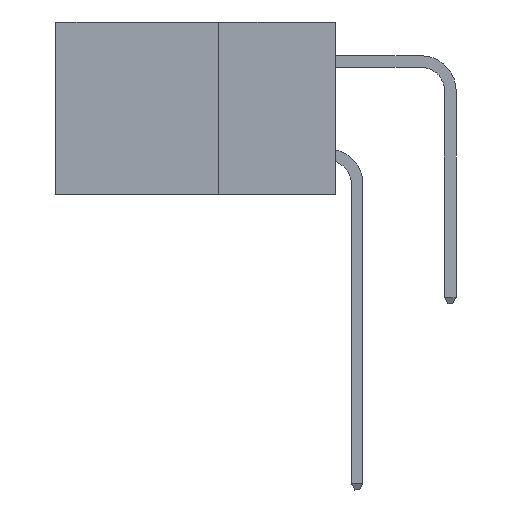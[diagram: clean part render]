
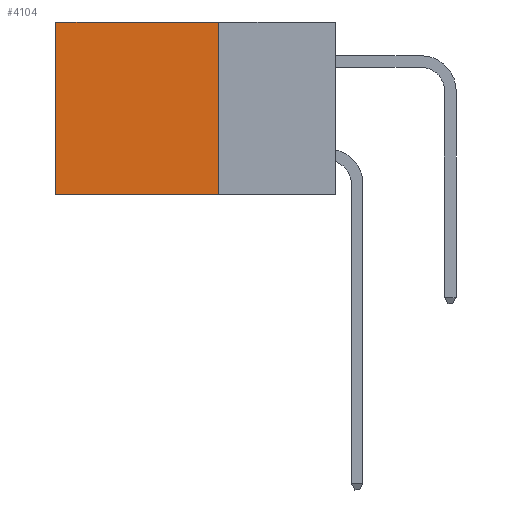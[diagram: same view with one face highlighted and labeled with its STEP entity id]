
A CAD part, left-side view. The second image highlights one B-rep face of the part: STEP entity #4104.
In plain terms, the highlighted planar face has unit normal (-1, 0, 0).
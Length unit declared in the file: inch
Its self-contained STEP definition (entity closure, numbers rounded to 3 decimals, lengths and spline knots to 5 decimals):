
#540 = VECTOR ( 'NONE', #29940, 39.37008 ) ;
#1571 = CARTESIAN_POINT ( 'NONE',  ( 0.2875, 0.6, 0. ) ) ;
#2058 = EDGE_CURVE ( 'NONE', #17198, #26423, #15869, .T. ) ;
#2449 = EDGE_CURVE ( 'NONE', #6529, #19729, #22710, .T. ) ;
#3277 = LINE ( 'NONE', #14994, #25613 ) ;
#4104 = ADVANCED_FACE ( 'NONE', ( #24076 ), #5557, .F. ) ;
#5557 = PLANE ( 'NONE',  #20178 ) ;
#6148 = CARTESIAN_POINT ( 'NONE',  ( 0.2875, 0.6, -0.37 ) ) ;
#6529 = VERTEX_POINT ( 'NONE', #15092 ) ;
#7688 = DIRECTION ( 'NONE',  ( 0., 1., 0. ) ) ;
#9575 = EDGE_CURVE ( 'NONE', #17198, #6529, #24203, .T. ) ;
#9994 = CARTESIAN_POINT ( 'NONE',  ( 0.2875, 0.25, 0. ) ) ;
#10143 = VECTOR ( 'NONE', #15763, 39.37008 ) ;
#14994 = CARTESIAN_POINT ( 'NONE',  ( 0.2875, 0.25, -0.37 ) ) ;
#15092 = CARTESIAN_POINT ( 'NONE',  ( 0.2875, 0.6, 0. ) ) ;
#15287 = DIRECTION ( 'NONE',  ( 0., 0., -1. ) ) ;
#15763 = DIRECTION ( 'NONE',  ( 0., 0., -1. ) ) ;
#15869 = LINE ( 'NONE', #30249, #540 ) ;
#16645 = CARTESIAN_POINT ( 'NONE',  ( 0.2875, 0.25, -0.37 ) ) ;
#17060 = EDGE_LOOP ( 'NONE', ( #27308, #19887, #30194, #21604 ) ) ;
#17198 = VERTEX_POINT ( 'NONE', #26461 ) ;
#19729 = VERTEX_POINT ( 'NONE', #6148 ) ;
#19887 = ORIENTED_EDGE ( 'NONE', *, *, #22315, .F. ) ;
#20055 = CARTESIAN_POINT ( 'NONE',  ( 0.2875, 0.25, 0. ) ) ;
#20178 = AXIS2_PLACEMENT_3D ( 'NONE', #20055, #22378, #15287 ) ;
#21604 = ORIENTED_EDGE ( 'NONE', *, *, #9575, .T. ) ;
#22315 = EDGE_CURVE ( 'NONE', #26423, #19729, #3277, .T. ) ;
#22378 = DIRECTION ( 'NONE',  ( 1., 0., 0. ) ) ;
#22710 = LINE ( 'NONE', #1571, #10143 ) ;
#24076 = FACE_OUTER_BOUND ( 'NONE', #17060, .T. ) ;
#24203 = LINE ( 'NONE', #9994, #27659 ) ;
#25613 = VECTOR ( 'NONE', #26261, 39.37008 ) ;
#26261 = DIRECTION ( 'NONE',  ( 0., 1., 0. ) ) ;
#26423 = VERTEX_POINT ( 'NONE', #16645 ) ;
#26461 = CARTESIAN_POINT ( 'NONE',  ( 0.2875, 0.25, 0. ) ) ;
#27308 = ORIENTED_EDGE ( 'NONE', *, *, #2449, .T. ) ;
#27659 = VECTOR ( 'NONE', #7688, 39.37008 ) ;
#29940 = DIRECTION ( 'NONE',  ( 0., 0., -1. ) ) ;
#30194 = ORIENTED_EDGE ( 'NONE', *, *, #2058, .F. ) ;
#30249 = CARTESIAN_POINT ( 'NONE',  ( 0.2875, 0.25, 0. ) ) ;
